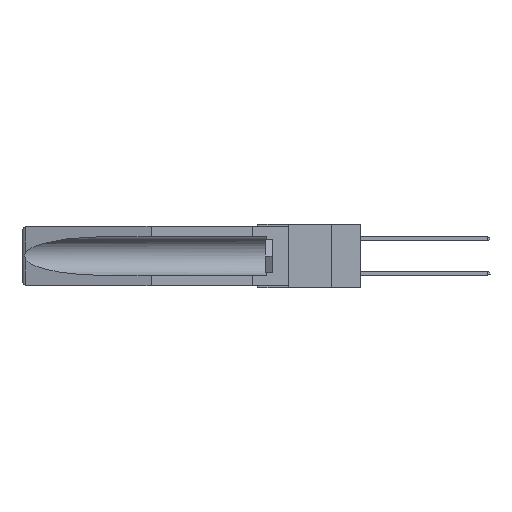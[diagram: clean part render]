
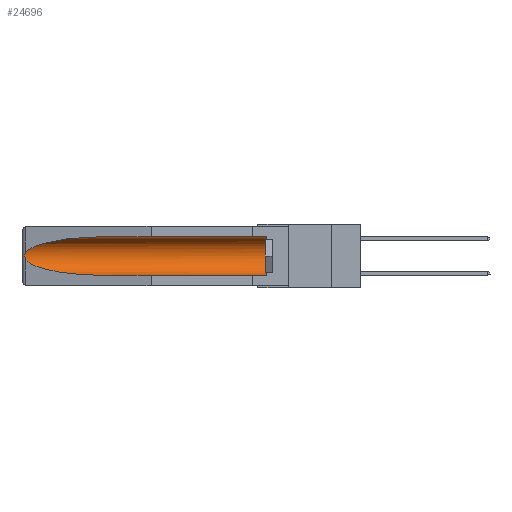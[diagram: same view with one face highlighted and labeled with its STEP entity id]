
A CAD part, left-side view. The second image highlights one B-rep face of the part: STEP entity #24696.
In plain terms, the highlighted cylindrical face has radius 2.857 mm (diameter 5.715 mm), a partial arc.
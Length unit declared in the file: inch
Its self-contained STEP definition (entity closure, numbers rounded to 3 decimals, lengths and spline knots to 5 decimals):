
#144 = EDGE_LOOP ( 'NONE', ( #14935, #14149, #19962, #20886, #3633, #18307 ) ) ;
#346 = CARTESIAN_POINT ( 'NONE',  ( 0.155, 1.07973, -0.059 ) ) ;
#843 = VERTEX_POINT ( 'NONE', #23122 ) ;
#1119 = CYLINDRICAL_SURFACE ( 'NONE', #4119, 0.1125 ) ;
#2104 = DIRECTION ( 'NONE',  ( 0., 1., 0. ) ) ;
#3127 = CARTESIAN_POINT ( 'NONE',  ( 0.25451, 1.48313, -0.24835 ) ) ;
#3415 = DIRECTION ( 'NONE',  ( 0., 0., 1. ) ) ;
#3633 = ORIENTED_EDGE ( 'NONE', *, *, #25363, .T. ) ;
#3971 = CARTESIAN_POINT ( 'NONE',  ( 0.26537, 1.52718, -0.14972 ) ) ;
#4119 = AXIS2_PLACEMENT_3D ( 'NONE', #7825, #12127, #14278 ) ;
#4366 = B_SPLINE_CURVE_WITH_KNOTS ( 'NONE', 3,
 ( #3971, #27667, #8225, #23222, #10361, #23971, #12536, #14676, #19007, #4604 ),
 .UNSPECIFIED., .F., .F.,
 ( 4, 2, 2, 2, 4 ),
 ( 0., 0.00029, 0.00058, 0.00087, 0.00117 ),
 .UNSPECIFIED. ) ;
#4604 = CARTESIAN_POINT ( 'NONE',  ( 0.26537, 1.52718, -0.19328 ) ) ;
#5424 = LINE ( 'NONE', #5891, #26277 ) ;
#5639 = LINE ( 'NONE', #10468, #27182 ) ;
#5891 = CARTESIAN_POINT ( 'NONE',  ( 0.155, -0.30754, -0.284 ) ) ;
#6374 = CARTESIAN_POINT ( 'NONE',  ( 0.155, 1.07973, -0.284 ) ) ;
#6562 = CARTESIAN_POINT ( 'NONE',  ( 0.155, 1.07973, -0.059 ) ) ;
#7527 = FACE_OUTER_BOUND ( 'NONE', #144, .T. ) ;
#7539 = CARTESIAN_POINT ( 'NONE',  ( 0.155, 0.126, -0.1715 ) ) ;
#7637 = VERTEX_POINT ( 'NONE', #8385 ) ;
#7825 = CARTESIAN_POINT ( 'NONE',  ( 0.155, -0.30754, -0.1715 ) ) ;
#8225 = CARTESIAN_POINT ( 'NONE',  ( 0.26654, 1.53092, -0.15636 ) ) ;
#8385 = CARTESIAN_POINT ( 'NONE',  ( 0.26537, 1.52718, -0.14972 ) ) ;
#9366 = CARTESIAN_POINT ( 'NONE',  ( 0.25451, 1.48313, -0.09465 ) ) ;
#9604 = CARTESIAN_POINT ( 'NONE',  ( 0.21114, 1.30732, -0.284 ) ) ;
#10361 = CARTESIAN_POINT ( 'NONE',  ( 0.2675, 1.53308, -0.16763 ) ) ;
#10468 = CARTESIAN_POINT ( 'NONE',  ( 0.155, -0.30754, -0.059 ) ) ;
#10773 = AXIS2_PLACEMENT_3D ( 'NONE', #7539, #24827, #3415 ) ;
#11343 = CARTESIAN_POINT ( 'NONE',  ( 0.21114, 1.30732, -0.059 ) ) ;
#12127 = DIRECTION ( 'NONE',  ( 0., 1., 0. ) ) ;
#12536 = CARTESIAN_POINT ( 'NONE',  ( 0.2673, 1.53269, -0.17917 ) ) ;
#12696 = EDGE_CURVE ( 'NONE', #7637, #843, #4366, .T. ) ;
#14149 = ORIENTED_EDGE ( 'NONE', *, *, #12696, .T. ) ;
#14278 = DIRECTION ( 'NONE',  ( 0., 0., 1. ) ) ;
#14493 = VERTEX_POINT ( 'NONE', #6562 ) ;
#14676 = CARTESIAN_POINT ( 'NONE',  ( 0.26655, 1.53094, -0.18657 ) ) ;
#14871 =( BOUNDED_CURVE ( )  B_SPLINE_CURVE ( 3, ( #26710, #3127, #9604, #24641 ),
 .UNSPECIFIED., .F., .F. ) 
 B_SPLINE_CURVE_WITH_KNOTS ( ( 4, 4 ),
 ( 0.1948, 1.5708 ),
 .UNSPECIFIED. ) 
 CURVE ( )  GEOMETRIC_REPRESENTATION_ITEM ( )  RATIONAL_B_SPLINE_CURVE ( ( 1., 0.848, 0.848, 1. ) ) 
 REPRESENTATION_ITEM ( '' )  );
#14935 = ORIENTED_EDGE ( 'NONE', *, *, #19424, .T. ) ;
#14946 = VERTEX_POINT ( 'NONE', #21190 ) ;
#15006 = EDGE_CURVE ( 'NONE', #14946, #26031, #5424, .T. ) ;
#15843 = CARTESIAN_POINT ( 'NONE',  ( 0.26537, 1.52718, -0.14972 ) ) ;
#17650 = VERTEX_POINT ( 'NONE', #24421 ) ;
#18307 = ORIENTED_EDGE ( 'NONE', *, *, #23390, .T. ) ;
#19007 = CARTESIAN_POINT ( 'NONE',  ( 0.26597, 1.5296, -0.19026 ) ) ;
#19424 = EDGE_CURVE ( 'NONE', #14493, #7637, #27303, .T. ) ;
#19910 = CIRCLE ( 'NONE', #10773, 0.1125 ) ;
#19962 = ORIENTED_EDGE ( 'NONE', *, *, #25402, .T. ) ;
#20886 = ORIENTED_EDGE ( 'NONE', *, *, #15006, .F. ) ;
#20900 = DIRECTION ( 'NONE',  ( 0., 1., 0. ) ) ;
#21190 = CARTESIAN_POINT ( 'NONE',  ( 0.155, 0.126, -0.284 ) ) ;
#23122 = CARTESIAN_POINT ( 'NONE',  ( 0.26537, 1.52718, -0.19328 ) ) ;
#23222 = CARTESIAN_POINT ( 'NONE',  ( 0.2673, 1.5327, -0.16383 ) ) ;
#23390 = EDGE_CURVE ( 'NONE', #17650, #14493, #5639, .T. ) ;
#23971 = CARTESIAN_POINT ( 'NONE',  ( 0.2675, 1.53308, -0.17534 ) ) ;
#24421 = CARTESIAN_POINT ( 'NONE',  ( 0.155, 0.126, -0.059 ) ) ;
#24641 = CARTESIAN_POINT ( 'NONE',  ( 0.155, 1.07973, -0.284 ) ) ;
#24696 = ADVANCED_FACE ( 'NONE', ( #7527 ), #1119, .F. ) ;
#24827 = DIRECTION ( 'NONE',  ( 0., -1., 0. ) ) ;
#25363 = EDGE_CURVE ( 'NONE', #14946, #17650, #19910, .T. ) ;
#25402 = EDGE_CURVE ( 'NONE', #843, #26031, #14871, .T. ) ;
#26031 = VERTEX_POINT ( 'NONE', #6374 ) ;
#26277 = VECTOR ( 'NONE', #20900, 39.37008 ) ;
#26710 = CARTESIAN_POINT ( 'NONE',  ( 0.26537, 1.52718, -0.19328 ) ) ;
#27182 = VECTOR ( 'NONE', #2104, 39.37008 ) ;
#27303 =( BOUNDED_CURVE ( )  B_SPLINE_CURVE ( 3, ( #346, #11343, #9366, #15843 ),
 .UNSPECIFIED., .F., .F. ) 
 B_SPLINE_CURVE_WITH_KNOTS ( ( 4, 4 ),
 ( 4.71239, 6.08839 ),
 .UNSPECIFIED. ) 
 CURVE ( )  GEOMETRIC_REPRESENTATION_ITEM ( )  RATIONAL_B_SPLINE_CURVE ( ( 1., 0.848, 0.848, 1. ) ) 
 REPRESENTATION_ITEM ( '' )  );
#27667 = CARTESIAN_POINT ( 'NONE',  ( 0.26597, 1.52961, -0.15275 ) ) ;
